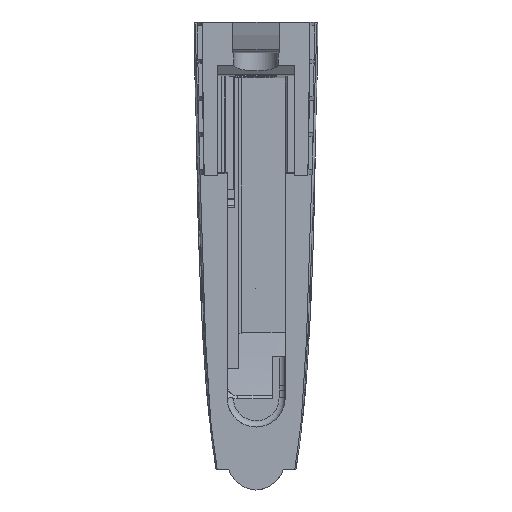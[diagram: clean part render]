
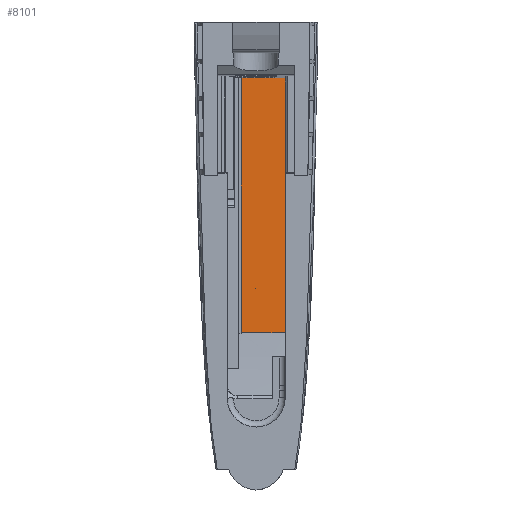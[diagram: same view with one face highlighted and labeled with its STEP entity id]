
A CAD part, front view. The second image highlights one B-rep face of the part: STEP entity #8101.
In plain terms, the highlighted planar face has unit normal (0, -1, 0).
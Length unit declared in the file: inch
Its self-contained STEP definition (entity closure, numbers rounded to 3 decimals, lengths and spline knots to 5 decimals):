
#320 = CARTESIAN_POINT ( 'NONE',  ( 1.104, 2.058, -5.68815 ) ) ;
#880 = DIRECTION ( 'NONE',  ( 0., 0., -1. ) ) ;
#937 = EDGE_CURVE ( 'NONE', #3582, #21313, #14882, .T. ) ;
#2221 = DIRECTION ( 'NONE',  ( -1., 0., 0. ) ) ;
#2532 = EDGE_CURVE ( 'NONE', #23394, #13550, #25920, .T. ) ;
#3582 = VERTEX_POINT ( 'NONE', #7620 ) ;
#7620 = CARTESIAN_POINT ( 'NONE',  ( 1.104, 2.058, -1.54785 ) ) ;
#8101 = ADVANCED_FACE ( 'NONE', ( #12545 ), #17517, .F. ) ;
#8423 = ORIENTED_EDGE ( 'NONE', *, *, #30528, .T. ) ;
#9352 = CARTESIAN_POINT ( 'NONE',  ( 0.39317, 2.058, -1.54785 ) ) ;
#10485 = DIRECTION ( 'NONE',  ( -1., 0., 0. ) ) ;
#12545 = FACE_OUTER_BOUND ( 'NONE', #26067, .T. ) ;
#13550 = VERTEX_POINT ( 'NONE', #29256 ) ;
#13823 = ORIENTED_EDGE ( 'NONE', *, *, #937, .T. ) ;
#14711 = CARTESIAN_POINT ( 'NONE',  ( 1.104, 2.058, -1.54785 ) ) ;
#14882 = LINE ( 'NONE', #24988, #15108 ) ;
#15108 = VECTOR ( 'NONE', #2221, 39.37008 ) ;
#16308 = EDGE_CURVE ( 'NONE', #3582, #23394, #23823, .T. ) ;
#16487 = VECTOR ( 'NONE', #19502, 39.37008 ) ;
#17245 = VECTOR ( 'NONE', #10485, 39.37008 ) ;
#17517 = PLANE ( 'NONE',  #28480 ) ;
#18760 = ORIENTED_EDGE ( 'NONE', *, *, #2532, .F. ) ;
#19021 = CARTESIAN_POINT ( 'NONE',  ( 1.104, 2.058, -1.54785 ) ) ;
#19502 = DIRECTION ( 'NONE',  ( 0., 0., -1. ) ) ;
#19714 = CARTESIAN_POINT ( 'NONE',  ( 1.104, 2.058, -5.68815 ) ) ;
#21313 = VERTEX_POINT ( 'NONE', #31869 ) ;
#22335 = DIRECTION ( 'NONE',  ( 0., 1., 0. ) ) ;
#22661 = DIRECTION ( 'NONE',  ( 0., 0., 1. ) ) ;
#23394 = VERTEX_POINT ( 'NONE', #19714 ) ;
#23823 = LINE ( 'NONE', #19021, #26166 ) ;
#24988 = CARTESIAN_POINT ( 'NONE',  ( 1.104, 2.058, -1.54785 ) ) ;
#25920 = LINE ( 'NONE', #320, #17245 ) ;
#26067 = EDGE_LOOP ( 'NONE', ( #8423, #18760, #28824, #13823 ) ) ;
#26166 = VECTOR ( 'NONE', #880, 39.37008 ) ;
#27126 = LINE ( 'NONE', #9352, #16487 ) ;
#28480 = AXIS2_PLACEMENT_3D ( 'NONE', #14711, #22335, #22661 ) ;
#28824 = ORIENTED_EDGE ( 'NONE', *, *, #16308, .F. ) ;
#29256 = CARTESIAN_POINT ( 'NONE',  ( 0.39317, 2.058, -5.68815 ) ) ;
#30528 = EDGE_CURVE ( 'NONE', #21313, #13550, #27126, .T. ) ;
#31869 = CARTESIAN_POINT ( 'NONE',  ( 0.39317, 2.058, -1.54785 ) ) ;
